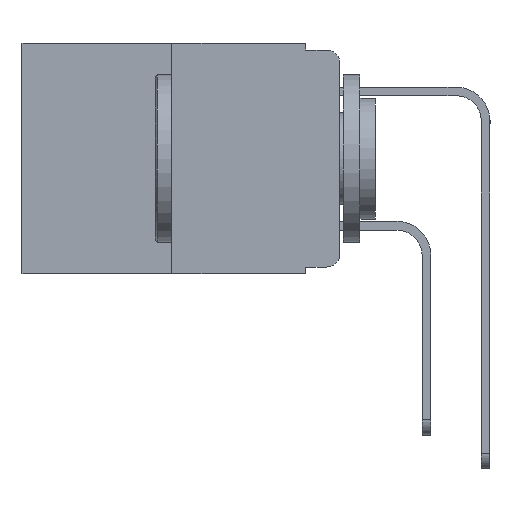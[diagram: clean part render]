
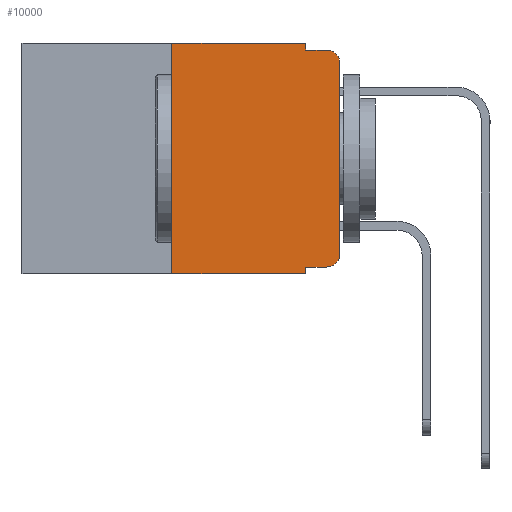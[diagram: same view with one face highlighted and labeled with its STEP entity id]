
A CAD part, left-side view. The second image highlights one B-rep face of the part: STEP entity #10000.
In plain terms, the highlighted planar face has unit normal (-1, 0, 0).
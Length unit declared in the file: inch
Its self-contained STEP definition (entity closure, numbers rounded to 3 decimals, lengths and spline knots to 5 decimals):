
#78 = VERTEX_POINT ( 'NONE', #4288 ) ;
#358 = ORIENTED_EDGE ( 'NONE', *, *, #2535, .F. ) ;
#431 = DIRECTION ( 'NONE',  ( 0., -1., 0. ) ) ;
#587 = ORIENTED_EDGE ( 'NONE', *, *, #4780, .T. ) ;
#644 = DIRECTION ( 'NONE',  ( -1., 0., 0. ) ) ;
#757 = ORIENTED_EDGE ( 'NONE', *, *, #6306, .T. ) ;
#909 = VERTEX_POINT ( 'NONE', #5137 ) ;
#1069 = CARTESIAN_POINT ( 'NONE',  ( 0., 0.02, -0.01 ) ) ;
#1131 = VECTOR ( 'NONE', #7679, 39.37008 ) ;
#2103 = CARTESIAN_POINT ( 'NONE',  ( 0., 0.473, 0. ) ) ;
#2234 = LINE ( 'NONE', #4915, #10444 ) ;
#2535 = EDGE_CURVE ( 'NONE', #11876, #9337, #10405, .T. ) ;
#2538 = ORIENTED_EDGE ( 'NONE', *, *, #10942, .T. ) ;
#2940 = VECTOR ( 'NONE', #6998, 39.37008 ) ;
#2989 = LINE ( 'NONE', #13563, #2940 ) ;
#3054 = CARTESIAN_POINT ( 'NONE',  ( 0., 0., -0.03 ) ) ;
#3071 = ORIENTED_EDGE ( 'NONE', *, *, #13916, .F. ) ;
#3192 = CIRCLE ( 'NONE', #6621, 0.02 ) ;
#3876 = LINE ( 'NONE', #6184, #6859 ) ;
#4132 = CARTESIAN_POINT ( 'NONE',  ( 0., 0.051, -0.333 ) ) ;
#4288 = CARTESIAN_POINT ( 'NONE',  ( 0., 0., -0.313 ) ) ;
#4363 = CARTESIAN_POINT ( 'NONE',  ( 0., 0.25, 0. ) ) ;
#4377 = PLANE ( 'NONE',  #11942 ) ;
#4614 = VERTEX_POINT ( 'NONE', #6579 ) ;
#4780 = EDGE_CURVE ( 'NONE', #13211, #9337, #3192, .T. ) ;
#4822 = ORIENTED_EDGE ( 'NONE', *, *, #8816, .T. ) ;
#4915 = CARTESIAN_POINT ( 'NONE',  ( 0., 0.473, 0. ) ) ;
#5137 = CARTESIAN_POINT ( 'NONE',  ( 0., 0.051, 0. ) ) ;
#5343 = CARTESIAN_POINT ( 'NONE',  ( 0., 0.02, -0.333 ) ) ;
#5812 = VECTOR ( 'NONE', #13940, 39.37008 ) ;
#6154 = LINE ( 'NONE', #11779, #5812 ) ;
#6184 = CARTESIAN_POINT ( 'NONE',  ( 0., 0.473, -0.343 ) ) ;
#6306 = EDGE_CURVE ( 'NONE', #78, #13211, #2989, .T. ) ;
#6576 = EDGE_CURVE ( 'NONE', #12001, #78, #9094, .T. ) ;
#6579 = CARTESIAN_POINT ( 'NONE',  ( 0., 0.25, -0.343 ) ) ;
#6621 = AXIS2_PLACEMENT_3D ( 'NONE', #7384, #14257, #13589 ) ;
#6649 = DIRECTION ( 'NONE',  ( 0., 0., -1. ) ) ;
#6859 = VECTOR ( 'NONE', #13841, 39.37008 ) ;
#6874 = DIRECTION ( 'NONE',  ( 0., -1., 0. ) ) ;
#6998 = DIRECTION ( 'NONE',  ( 0., 0., 1. ) ) ;
#7293 = CARTESIAN_POINT ( 'NONE',  ( 0., 0.051, -0.01 ) ) ;
#7384 = CARTESIAN_POINT ( 'NONE',  ( 0., 0.02, -0.03 ) ) ;
#7385 = CARTESIAN_POINT ( 'NONE',  ( 0., 0.02, -0.313 ) ) ;
#7625 = ORIENTED_EDGE ( 'NONE', *, *, #12479, .F. ) ;
#7679 = DIRECTION ( 'NONE',  ( 0., 0., -1. ) ) ;
#7932 = AXIS2_PLACEMENT_3D ( 'NONE', #7385, #644, #8508 ) ;
#8050 = DIRECTION ( 'NONE',  ( 0., -1., 0. ) ) ;
#8508 = DIRECTION ( 'NONE',  ( 0., 0., -1. ) ) ;
#8578 = LINE ( 'NONE', #10520, #14022 ) ;
#8816 = EDGE_CURVE ( 'NONE', #10400, #12001, #12596, .T. ) ;
#9094 = CIRCLE ( 'NONE', #7932, 0.02 ) ;
#9337 = VERTEX_POINT ( 'NONE', #1069 ) ;
#9377 = LINE ( 'NONE', #14215, #1131 ) ;
#9679 = VECTOR ( 'NONE', #6874, 39.37008 ) ;
#9867 = ORIENTED_EDGE ( 'NONE', *, *, #12987, .F. ) ;
#9902 = CARTESIAN_POINT ( 'NONE',  ( 0., 0.051, -0.343 ) ) ;
#10000 = ADVANCED_FACE ( 'NONE', ( #12737 ), #4377, .F. ) ;
#10073 = VECTOR ( 'NONE', #8050, 39.37008 ) ;
#10400 = VERTEX_POINT ( 'NONE', #4132 ) ;
#10405 = LINE ( 'NONE', #13213, #10073 ) ;
#10444 = VECTOR ( 'NONE', #431, 39.37008 ) ;
#10520 = CARTESIAN_POINT ( 'NONE',  ( 0., 0.25, 0. ) ) ;
#10543 = VERTEX_POINT ( 'NONE', #4363 ) ;
#10942 = EDGE_CURVE ( 'NONE', #4614, #13927, #3876, .T. ) ;
#11021 = EDGE_CURVE ( 'NONE', #10400, #13927, #6154, .T. ) ;
#11779 = CARTESIAN_POINT ( 'NONE',  ( 0., 0.051, 0. ) ) ;
#11876 = VERTEX_POINT ( 'NONE', #7293 ) ;
#11942 = AXIS2_PLACEMENT_3D ( 'NONE', #2103, #13244, #6649 ) ;
#12001 = VERTEX_POINT ( 'NONE', #5343 ) ;
#12030 = EDGE_LOOP ( 'NONE', ( #757, #587, #358, #3071, #9867, #7625, #2538, #12915, #4822, #13937 ) ) ;
#12479 = EDGE_CURVE ( 'NONE', #4614, #10543, #8578, .T. ) ;
#12596 = LINE ( 'NONE', #13404, #9679 ) ;
#12737 = FACE_OUTER_BOUND ( 'NONE', #12030, .T. ) ;
#12915 = ORIENTED_EDGE ( 'NONE', *, *, #11021, .F. ) ;
#12987 = EDGE_CURVE ( 'NONE', #10543, #909, #2234, .T. ) ;
#13211 = VERTEX_POINT ( 'NONE', #3054 ) ;
#13213 = CARTESIAN_POINT ( 'NONE',  ( 0., 0.051, -0.01 ) ) ;
#13244 = DIRECTION ( 'NONE',  ( 1., 0., 0. ) ) ;
#13404 = CARTESIAN_POINT ( 'NONE',  ( 0., 0.051, -0.333 ) ) ;
#13563 = CARTESIAN_POINT ( 'NONE',  ( 0., 0., 0. ) ) ;
#13589 = DIRECTION ( 'NONE',  ( 0., 0., -1. ) ) ;
#13784 = DIRECTION ( 'NONE',  ( 0., 0., 1. ) ) ;
#13841 = DIRECTION ( 'NONE',  ( 0., -1., 0. ) ) ;
#13916 = EDGE_CURVE ( 'NONE', #909, #11876, #9377, .T. ) ;
#13927 = VERTEX_POINT ( 'NONE', #9902 ) ;
#13937 = ORIENTED_EDGE ( 'NONE', *, *, #6576, .T. ) ;
#13940 = DIRECTION ( 'NONE',  ( 0., 0., -1. ) ) ;
#14022 = VECTOR ( 'NONE', #13784, 39.37008 ) ;
#14215 = CARTESIAN_POINT ( 'NONE',  ( 0., 0.051, 0. ) ) ;
#14257 = DIRECTION ( 'NONE',  ( -1., 0., 0. ) ) ;
